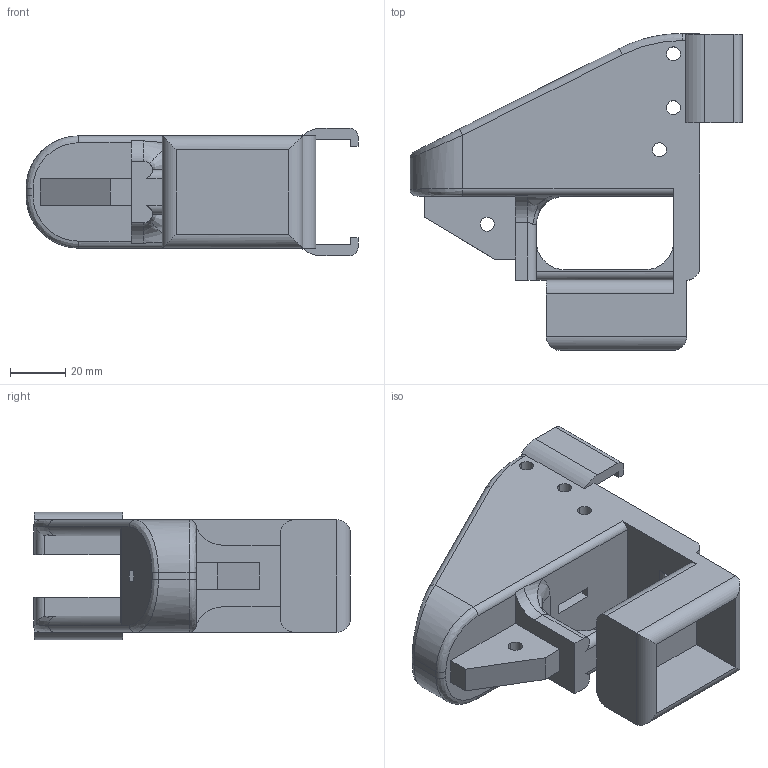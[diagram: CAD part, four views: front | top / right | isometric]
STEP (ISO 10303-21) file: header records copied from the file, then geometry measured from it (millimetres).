
FILE_DESCRIPTION (( 'STEP AP214' ), '1' );
FILE_NAME ('cerberusframe.STEP', '2013-07-13T20:17:17', ( '' ), ( '' ), 'SwSTEP 2.0', 'SolidWorks 2013', '' );
FILE_SCHEMA (( 'AUTOMOTIVE_DESIGN' ));
Length unit declared in the file: millimetre
Products named in the file (1): cerberusframe
Bounding box: 120.18 x 114.71 x 46.1 mm (x, y, z)
Volume: 145736.4 mm3; surface area: 48293.9 mm2
Topology: 1 solids, 1 shells, 266 faces, 728 edges, 472 vertices
Faces by surface type: plane 150, bspline 62, cylinder 54
Entity records: 12978 total; most frequent: CARTESIAN_POINT 5191, ORIENTED_EDGE 1456, DIRECTION 1112, EDGE_CURVE 728, LINE 498, VECTOR 498, VERTEX_POINT 472, AXIS2_PLACEMENT_3D 307
